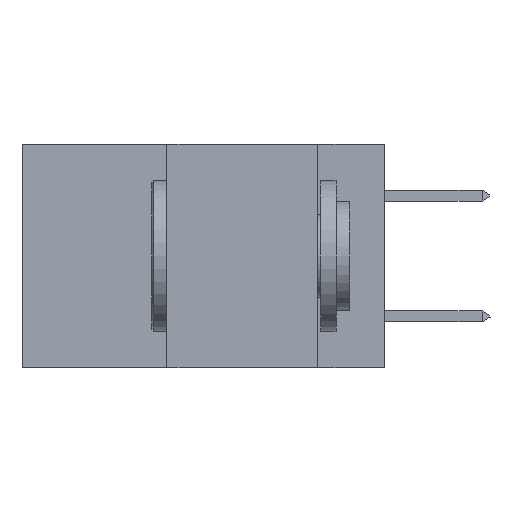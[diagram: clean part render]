
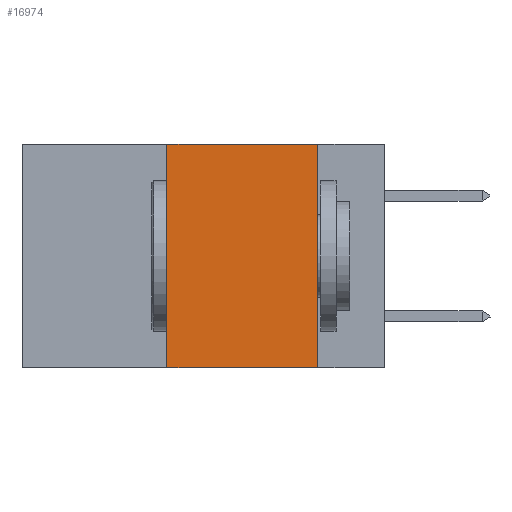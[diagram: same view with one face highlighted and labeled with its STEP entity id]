
A CAD part, left-side view. The second image highlights one B-rep face of the part: STEP entity #16974.
In plain terms, the highlighted planar face has unit normal (-1, 0, 0).
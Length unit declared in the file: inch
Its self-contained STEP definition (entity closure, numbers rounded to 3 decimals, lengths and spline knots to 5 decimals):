
#716 = VECTOR ( 'NONE', #22325, 39.37008 ) ;
#802 = VERTEX_POINT ( 'NONE', #17169 ) ;
#810 = VECTOR ( 'NONE', #21058, 39.37008 ) ;
#1465 = CARTESIAN_POINT ( 'NONE',  ( 0., 0.36, 0. ) ) ;
#2211 = CARTESIAN_POINT ( 'NONE',  ( 0., 0.6, -0.37 ) ) ;
#2999 = EDGE_CURVE ( 'NONE', #802, #11633, #15707, .T. ) ;
#4196 = DIRECTION ( 'NONE',  ( 1., 0., 0. ) ) ;
#5622 = CARTESIAN_POINT ( 'NONE',  ( 0., 0.6, 0. ) ) ;
#6115 = DIRECTION ( 'NONE',  ( 0., 0., -1. ) ) ;
#8291 = EDGE_LOOP ( 'NONE', ( #11242, #12301, #9864, #9247 ) ) ;
#8560 = LINE ( 'NONE', #10170, #9733 ) ;
#9247 = ORIENTED_EDGE ( 'NONE', *, *, #2999, .T. ) ;
#9733 = VECTOR ( 'NONE', #23293, 39.37008 ) ;
#9801 = PLANE ( 'NONE',  #22185 ) ;
#9864 = ORIENTED_EDGE ( 'NONE', *, *, #15614, .F. ) ;
#10170 = CARTESIAN_POINT ( 'NONE',  ( 0., 0.36, 0. ) ) ;
#11242 = ORIENTED_EDGE ( 'NONE', *, *, #21815, .F. ) ;
#11633 = VERTEX_POINT ( 'NONE', #22038 ) ;
#12301 = ORIENTED_EDGE ( 'NONE', *, *, #22644, .F. ) ;
#12321 = CARTESIAN_POINT ( 'NONE',  ( 0., 0.11, 0. ) ) ;
#13838 = VERTEX_POINT ( 'NONE', #1465 ) ;
#15570 = CARTESIAN_POINT ( 'NONE',  ( 0., 0.6, 0. ) ) ;
#15614 = EDGE_CURVE ( 'NONE', #802, #13838, #8560, .T. ) ;
#15707 = LINE ( 'NONE', #2211, #810 ) ;
#16392 = CARTESIAN_POINT ( 'NONE',  ( 0., 0.11, 0. ) ) ;
#16974 = ADVANCED_FACE ( 'NONE', ( #21321 ), #9801, .F. ) ;
#17169 = CARTESIAN_POINT ( 'NONE',  ( 0., 0.36, -0.37 ) ) ;
#18676 = LINE ( 'NONE', #16392, #716 ) ;
#18958 = DIRECTION ( 'NONE',  ( 0., -1., 0. ) ) ;
#19672 = VERTEX_POINT ( 'NONE', #12321 ) ;
#21058 = DIRECTION ( 'NONE',  ( 0., -1., 0. ) ) ;
#21321 = FACE_OUTER_BOUND ( 'NONE', #8291, .T. ) ;
#21574 = LINE ( 'NONE', #5622, #24332 ) ;
#21815 = EDGE_CURVE ( 'NONE', #19672, #11633, #18676, .T. ) ;
#22038 = CARTESIAN_POINT ( 'NONE',  ( 0., 0.11, -0.37 ) ) ;
#22185 = AXIS2_PLACEMENT_3D ( 'NONE', #15570, #4196, #6115 ) ;
#22325 = DIRECTION ( 'NONE',  ( 0., 0., -1. ) ) ;
#22644 = EDGE_CURVE ( 'NONE', #13838, #19672, #21574, .T. ) ;
#23293 = DIRECTION ( 'NONE',  ( 0., 0., 1. ) ) ;
#24332 = VECTOR ( 'NONE', #18958, 39.37008 ) ;
